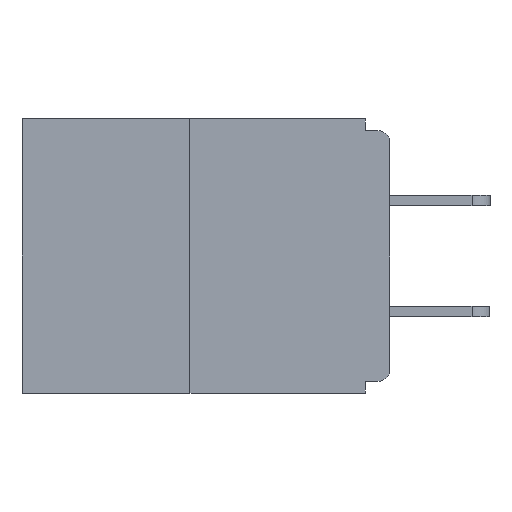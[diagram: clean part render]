
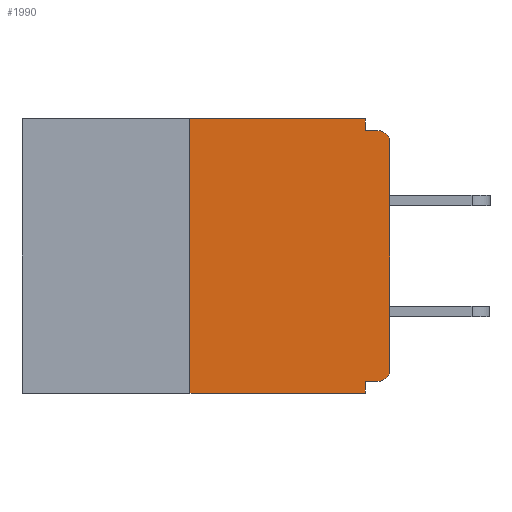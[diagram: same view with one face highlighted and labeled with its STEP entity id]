
A CAD part, left-side view. The second image highlights one B-rep face of the part: STEP entity #1990.
In plain terms, the highlighted planar face has unit normal (-1, 0, 0).
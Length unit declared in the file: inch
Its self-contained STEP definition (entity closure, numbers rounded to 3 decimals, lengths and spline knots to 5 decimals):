
#23 = DIRECTION ( 'NONE',  ( 0., 0., -1. ) ) ;
#249 = VERTEX_POINT ( 'NONE', #8031 ) ;
#581 = DIRECTION ( 'NONE',  ( 0., 0., 1. ) ) ;
#604 = VERTEX_POINT ( 'NONE', #18634 ) ;
#665 = ORIENTED_EDGE ( 'NONE', *, *, #2982, .T. ) ;
#938 = VECTOR ( 'NONE', #12048, 39.37008 ) ;
#1337 = CARTESIAN_POINT ( 'NONE',  ( 0., 0., -0.328 ) ) ;
#1523 = VECTOR ( 'NONE', #3057, 39.37008 ) ;
#1741 = DIRECTION ( 'NONE',  ( 0., 0., 1. ) ) ;
#1980 = CARTESIAN_POINT ( 'NONE',  ( 0., 0.015, -0.328 ) ) ;
#1990 = ADVANCED_FACE ( 'NONE', ( #16140 ), #14691, .F. ) ;
#1999 = VECTOR ( 'NONE', #20574, 39.37008 ) ;
#2060 = VECTOR ( 'NONE', #1741, 39.37008 ) ;
#2656 = ORIENTED_EDGE ( 'NONE', *, *, #3843, .T. ) ;
#2982 = EDGE_CURVE ( 'NONE', #11925, #6016, #17699, .T. ) ;
#3057 = DIRECTION ( 'NONE',  ( 0., 0., -1. ) ) ;
#3517 = DIRECTION ( 'NONE',  ( 0., -1., 0. ) ) ;
#3631 = VERTEX_POINT ( 'NONE', #14042 ) ;
#3739 = LINE ( 'NONE', #8231, #1523 ) ;
#3843 = EDGE_CURVE ( 'NONE', #604, #249, #10068, .T. ) ;
#4231 = EDGE_CURVE ( 'NONE', #9169, #11925, #21444, .T. ) ;
#4253 = CARTESIAN_POINT ( 'NONE',  ( 0., 0.46, 0. ) ) ;
#4598 = VECTOR ( 'NONE', #581, 39.37008 ) ;
#5653 = VECTOR ( 'NONE', #3517, 39.37008 ) ;
#5748 = VERTEX_POINT ( 'NONE', #1980 ) ;
#6016 = VERTEX_POINT ( 'NONE', #13267 ) ;
#6058 = DIRECTION ( 'NONE',  ( 0., 0., -1. ) ) ;
#6951 = CARTESIAN_POINT ( 'NONE',  ( 0., 0., -0.313 ) ) ;
#7224 = LINE ( 'NONE', #10495, #2060 ) ;
#7247 = LINE ( 'NONE', #22072, #14802 ) ;
#7385 = CARTESIAN_POINT ( 'NONE',  ( 0., 0.46, -0.343 ) ) ;
#7662 = DIRECTION ( 'NONE',  ( -1., 0., 0. ) ) ;
#8031 = CARTESIAN_POINT ( 'NONE',  ( 0., 0.031, -0.343 ) ) ;
#8074 = CARTESIAN_POINT ( 'NONE',  ( 0., 0.031, 0. ) ) ;
#8231 = CARTESIAN_POINT ( 'NONE',  ( 0., 0.031, 0. ) ) ;
#8941 = LINE ( 'NONE', #10414, #5653 ) ;
#8943 = CARTESIAN_POINT ( 'NONE',  ( 0., 0.015, -0.313 ) ) ;
#9040 = ORIENTED_EDGE ( 'NONE', *, *, #16124, .F. ) ;
#9169 = VERTEX_POINT ( 'NONE', #6951 ) ;
#9718 = VERTEX_POINT ( 'NONE', #8074 ) ;
#10068 = LINE ( 'NONE', #7385, #13845 ) ;
#10150 = AXIS2_PLACEMENT_3D ( 'NONE', #16293, #7662, #21552 ) ;
#10414 = CARTESIAN_POINT ( 'NONE',  ( 0., 0.46, 0. ) ) ;
#10495 = CARTESIAN_POINT ( 'NONE',  ( 0., 0.25, 0. ) ) ;
#10552 = AXIS2_PLACEMENT_3D ( 'NONE', #8943, #21081, #23 ) ;
#11167 = ORIENTED_EDGE ( 'NONE', *, *, #22181, .F. ) ;
#11369 = EDGE_LOOP ( 'NONE', ( #19367, #22103, #2656, #11167, #20459, #14659, #15411, #665, #21975, #9040 ) ) ;
#11925 = VERTEX_POINT ( 'NONE', #20466 ) ;
#12048 = DIRECTION ( 'NONE',  ( 0., -1., 0. ) ) ;
#12374 = CIRCLE ( 'NONE', #10552, 0.015 ) ;
#12489 = EDGE_CURVE ( 'NONE', #13335, #9718, #8941, .T. ) ;
#12625 = DIRECTION ( 'NONE',  ( 0., -1., 0. ) ) ;
#13267 = CARTESIAN_POINT ( 'NONE',  ( 0., 0.015, -0.015 ) ) ;
#13335 = VERTEX_POINT ( 'NONE', #15962 ) ;
#13681 = EDGE_CURVE ( 'NONE', #604, #13335, #7224, .T. ) ;
#13845 = VECTOR ( 'NONE', #12625, 39.37008 ) ;
#14042 = CARTESIAN_POINT ( 'NONE',  ( 0., 0.031, -0.015 ) ) ;
#14659 = ORIENTED_EDGE ( 'NONE', *, *, #17042, .T. ) ;
#14691 = PLANE ( 'NONE',  #18069 ) ;
#14802 = VECTOR ( 'NONE', #16828, 39.37008 ) ;
#15411 = ORIENTED_EDGE ( 'NONE', *, *, #4231, .T. ) ;
#15962 = CARTESIAN_POINT ( 'NONE',  ( 0., 0.25, 0. ) ) ;
#16124 = EDGE_CURVE ( 'NONE', #9718, #3631, #3739, .T. ) ;
#16140 = FACE_OUTER_BOUND ( 'NONE', #11369, .T. ) ;
#16293 = CARTESIAN_POINT ( 'NONE',  ( 0., 0.015, -0.03 ) ) ;
#16520 = DIRECTION ( 'NONE',  ( 1., 0., 0. ) ) ;
#16828 = DIRECTION ( 'NONE',  ( 0., 0., -1. ) ) ;
#16867 = EDGE_CURVE ( 'NONE', #3631, #6016, #17513, .T. ) ;
#17042 = EDGE_CURVE ( 'NONE', #5748, #9169, #12374, .T. ) ;
#17043 = CARTESIAN_POINT ( 'NONE',  ( 0., 0., -0.015 ) ) ;
#17513 = LINE ( 'NONE', #17043, #938 ) ;
#17699 = CIRCLE ( 'NONE', #10150, 0.015 ) ;
#18069 = AXIS2_PLACEMENT_3D ( 'NONE', #4253, #16520, #6058 ) ;
#18449 = EDGE_CURVE ( 'NONE', #5748, #21564, #21033, .T. ) ;
#18634 = CARTESIAN_POINT ( 'NONE',  ( 0., 0.25, -0.343 ) ) ;
#19367 = ORIENTED_EDGE ( 'NONE', *, *, #12489, .F. ) ;
#19520 = CARTESIAN_POINT ( 'NONE',  ( 0., 0.031, -0.328 ) ) ;
#19654 = CARTESIAN_POINT ( 'NONE',  ( 0., 0., 0. ) ) ;
#20459 = ORIENTED_EDGE ( 'NONE', *, *, #18449, .F. ) ;
#20466 = CARTESIAN_POINT ( 'NONE',  ( 0., 0., -0.03 ) ) ;
#20574 = DIRECTION ( 'NONE',  ( 0., 1., 0. ) ) ;
#21033 = LINE ( 'NONE', #1337, #1999 ) ;
#21081 = DIRECTION ( 'NONE',  ( -1., 0., 0. ) ) ;
#21444 = LINE ( 'NONE', #19654, #4598 ) ;
#21552 = DIRECTION ( 'NONE',  ( 0., 0., -1. ) ) ;
#21564 = VERTEX_POINT ( 'NONE', #19520 ) ;
#21975 = ORIENTED_EDGE ( 'NONE', *, *, #16867, .F. ) ;
#22072 = CARTESIAN_POINT ( 'NONE',  ( 0., 0.031, -0.343 ) ) ;
#22103 = ORIENTED_EDGE ( 'NONE', *, *, #13681, .F. ) ;
#22181 = EDGE_CURVE ( 'NONE', #21564, #249, #7247, .T. ) ;
